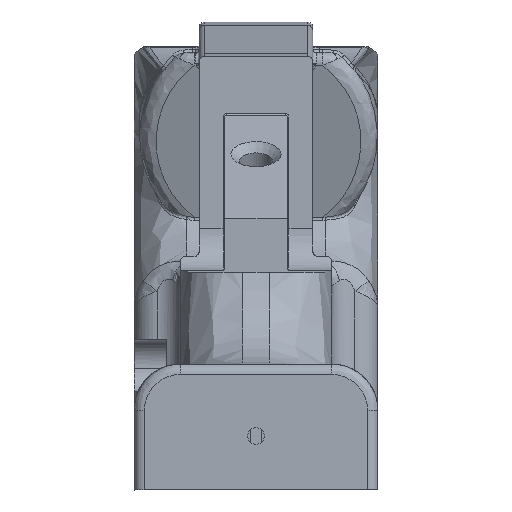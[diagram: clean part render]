
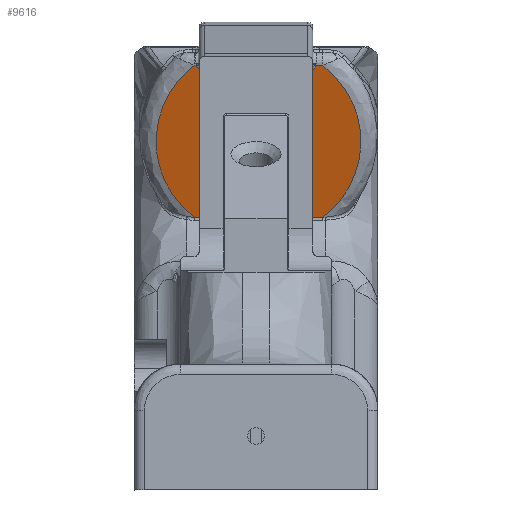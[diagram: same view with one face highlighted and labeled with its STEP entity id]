
A CAD part, left-side view. The second image highlights one B-rep face of the part: STEP entity #9616.
In plain terms, the highlighted face is planar.
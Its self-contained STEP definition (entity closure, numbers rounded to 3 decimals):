
#287 = CARTESIAN_POINT ( 'NONE',  ( -86.38, -58.957, 9.041 ) ) ;
#300 = VERTEX_POINT ( 'NONE', #3083 ) ;
#1211 = EDGE_CURVE ( 'NONE', #7501, #18581, #15948, .T. ) ;
#1220 = ORIENTED_EDGE ( 'NONE', *, *, #18913, .T. ) ;
#1431 = ORIENTED_EDGE ( 'NONE', *, *, #1211, .F. ) ;
#1519 = CARTESIAN_POINT ( 'NONE',  ( -79.11, -35.899, 9.385 ) ) ;
#1531 = CARTESIAN_POINT ( 'NONE',  ( -86.423, -59.093, 9.38 ) ) ;
#1605 = ORIENTED_EDGE ( 'NONE', *, *, #19267, .T. ) ;
#1767 = CARTESIAN_POINT ( 'NONE',  ( -81.144, -42.35, -18.578 ) ) ;
#1839 = ORIENTED_EDGE ( 'NONE', *, *, #10694, .T. ) ;
#1852 = CARTESIAN_POINT ( 'NONE',  ( -86.156, -58.248, 8.376 ) ) ;
#2007 = EDGE_CURVE ( 'NONE', #4205, #10850, #8191, .T. ) ;
#2132 = EDGE_CURVE ( 'NONE', #18581, #7602, #13308, .T. ) ;
#2375 = CARTESIAN_POINT ( 'NONE',  ( -86.342, -58.835, -8.976 ) ) ;
#2548 = B_SPLINE_CURVE_WITH_KNOTS ( 'NONE', 3,
 ( #3280, #13745, #6333, #15331, #7869, #15270, #1852, #18113, #18312, #12299, #3406, #9184, #13610, #13802, #287, #4910 ),
 .UNSPECIFIED., .F., .F.,
 ( 4, 1, 2, 2, 2, 1, 2, 2, 4 ),
 ( 0., 0.125, 0.188, 0.25, 0.5, 0.625, 0.688, 0.75, 1. ),
 .UNSPECIFIED. ) ;
#2953 = CARTESIAN_POINT ( 'NONE',  ( -86.423, -59.093, -3.161 ) ) ;
#3083 = CARTESIAN_POINT ( 'NONE',  ( -79.11, -35.899, -10.166 ) ) ;
#3268 = PLANE ( 'NONE',  #10192 ) ;
#3280 = CARTESIAN_POINT ( 'NONE',  ( -86.122, -58.139, 7.855 ) ) ;
#3406 = CARTESIAN_POINT ( 'NONE',  ( -86.267, -58.6, 8.817 ) ) ;
#3735 = CARTESIAN_POINT ( 'NONE',  ( -86.401, -59.025, -9.062 ) ) ;
#3867 = CARTESIAN_POINT ( 'NONE',  ( -86.191, -58.359, -8.556 ) ) ;
#4205 = VERTEX_POINT ( 'NONE', #8599 ) ;
#4249 = B_SPLINE_CURVE_WITH_KNOTS ( 'NONE', 3,
 ( #8255, #3735, #17134, #2375, #18641, #14331, #8319, #12756, #3867, #5366, #12882, #15653, #14268, #18699, #9691, #8459 ),
 .UNSPECIFIED., .F., .F.,
 ( 4, 1, 2, 2, 2, 1, 2, 2, 4 ),
 ( 0., 0.125, 0.187, 0.25, 0.5, 0.625, 0.687, 0.75, 1. ),
 .UNSPECIFIED. ) ;
#4419 = DIRECTION ( 'NONE',  ( 0., 0., -1. ) ) ;
#4565 = CARTESIAN_POINT ( 'NONE',  ( -86.423, -59.093, -0.39 ) ) ;
#4910 = CARTESIAN_POINT ( 'NONE',  ( -86.423, -59.093, 9.083 ) ) ;
#4961 = VECTOR ( 'NONE', #9032, 1000. ) ;
#5224 = CARTESIAN_POINT ( 'NONE',  ( -86.122, -58.139, -0.39 ) ) ;
#5366 = CARTESIAN_POINT ( 'NONE',  ( -86.173, -58.301, -8.467 ) ) ;
#6333 = CARTESIAN_POINT ( 'NONE',  ( -86.125, -58.147, 8.019 ) ) ;
#7501 = VERTEX_POINT ( 'NONE', #1519 ) ;
#7602 = VERTEX_POINT ( 'NONE', #18106 ) ;
#7869 = CARTESIAN_POINT ( 'NONE',  ( -86.136, -58.184, 8.18 ) ) ;
#8191 = LINE ( 'NONE', #5224, #18701 ) ;
#8206 = LINE ( 'NONE', #2953, #18248 ) ;
#8255 = CARTESIAN_POINT ( 'NONE',  ( -86.423, -59.093, -9.083 ) ) ;
#8319 = CARTESIAN_POINT ( 'NONE',  ( -86.266, -58.595, -8.823 ) ) ;
#8459 = CARTESIAN_POINT ( 'NONE',  ( -86.122, -58.139, -7.855 ) ) ;
#8599 = CARTESIAN_POINT ( 'NONE',  ( -86.122, -58.139, -7.855 ) ) ;
#8964 = EDGE_CURVE ( 'NONE', #11806, #15990, #8206, .T. ) ;
#9032 = DIRECTION ( 'NONE',  ( 0., 0., -1. ) ) ;
#9039 = CARTESIAN_POINT ( 'NONE',  ( -84.39, -52.645, -18.576 ) ) ;
#9184 = CARTESIAN_POINT ( 'NONE',  ( -86.285, -58.657, 8.862 ) ) ;
#9616 = ADVANCED_FACE ( 'NONE', ( #17098 ), #3268, .T. ) ;
#9691 = CARTESIAN_POINT ( 'NONE',  ( -86.122, -58.139, -7.988 ) ) ;
#10192 = AXIS2_PLACEMENT_3D ( 'NONE', #10394, #13596, #13666 ) ;
#10394 = CARTESIAN_POINT ( 'NONE',  ( -82.766, -47.494, -0.39 ) ) ;
#10685 = CARTESIAN_POINT ( 'NONE',  ( -79.11, -35.899, 9.385 ) ) ;
#10694 = EDGE_CURVE ( 'NONE', #10850, #7602, #2548, .T. ) ;
#10850 = VERTEX_POINT ( 'NONE', #12365 ) ;
#10875 = ORIENTED_EDGE ( 'NONE', *, *, #2132, .F. ) ;
#11022 = ORIENTED_EDGE ( 'NONE', *, *, #8964, .F. ) ;
#11806 = VERTEX_POINT ( 'NONE', #16046 ) ;
#12152 = DIRECTION ( 'NONE',  ( 0., 0., -1. ) ) ;
#12255 = CARTESIAN_POINT ( 'NONE',  ( -86.423, -59.093, 9.38 ) ) ;
#12299 = CARTESIAN_POINT ( 'NONE',  ( -86.242, -58.518, 8.747 ) ) ;
#12365 = CARTESIAN_POINT ( 'NONE',  ( -86.122, -58.139, 7.855 ) ) ;
#12509 = ORIENTED_EDGE ( 'NONE', *, *, #2007, .T. ) ;
#12756 = CARTESIAN_POINT ( 'NONE',  ( -86.233, -58.49, -8.725 ) ) ;
#12882 = CARTESIAN_POINT ( 'NONE',  ( -86.159, -58.255, -8.373 ) ) ;
#13308 = LINE ( 'NONE', #4565, #4961 ) ;
#13592 = CARTESIAN_POINT ( 'NONE',  ( -79.11, -35.899, -10.166 ) ) ;
#13596 = DIRECTION ( 'NONE',  ( -0.954, 0.301, 0. ) ) ;
#13610 = CARTESIAN_POINT ( 'NONE',  ( -86.295, -58.688, 8.885 ) ) ;
#13666 = DIRECTION ( 'NONE',  ( -0.301, -0.954, 0. ) ) ;
#13701 = CARTESIAN_POINT ( 'NONE',  ( -84.39, -52.645, 17.795 ) ) ;
#13745 = CARTESIAN_POINT ( 'NONE',  ( -86.122, -58.139, 7.921 ) ) ;
#13786 = CARTESIAN_POINT ( 'NONE',  ( -86.423, -59.093, -10.161 ) ) ;
#13802 = CARTESIAN_POINT ( 'NONE',  ( -86.34, -58.832, 8.982 ) ) ;
#13964 = EDGE_LOOP ( 'NONE', ( #15762, #11022, #1220, #12509, #1839, #10875, #1431, #1605 ) ) ;
#14268 = CARTESIAN_POINT ( 'NONE',  ( -86.146, -58.214, -8.275 ) ) ;
#14331 = CARTESIAN_POINT ( 'NONE',  ( -86.314, -58.747, -8.924 ) ) ;
#14340 = EDGE_CURVE ( 'NONE', #15990, #300, #17252, .T. ) ;
#15270 = CARTESIAN_POINT ( 'NONE',  ( -86.139, -58.192, 8.21 ) ) ;
#15331 = CARTESIAN_POINT ( 'NONE',  ( -86.131, -58.167, 8.116 ) ) ;
#15349 = CARTESIAN_POINT ( 'NONE',  ( -81.144, -42.35, 17.797 ) ) ;
#15653 = CARTESIAN_POINT ( 'NONE',  ( -86.15, -58.227, -8.309 ) ) ;
#15762 = ORIENTED_EDGE ( 'NONE', *, *, #14340, .F. ) ;
#15948 =( BOUNDED_CURVE ( )  B_SPLINE_CURVE ( 3, ( #10685, #15349, #13701, #12255 ),
 .UNSPECIFIED., .F., .T. ) 
 B_SPLINE_CURVE_WITH_KNOTS ( ( 4, 4 ),
 ( 0., 1. ),
 .UNSPECIFIED. ) 
 CURVE ( )  GEOMETRIC_REPRESENTATION_ITEM ( )  RATIONAL_B_SPLINE_CURVE ( ( 1., 0.751, 0.751, 1. ) ) 
 REPRESENTATION_ITEM ( '' )  );
#15990 = VERTEX_POINT ( 'NONE', #18988 ) ;
#16046 = CARTESIAN_POINT ( 'NONE',  ( -86.423, -59.093, -9.083 ) ) ;
#16542 = LINE ( 'NONE', #16602, #16761 ) ;
#16602 = CARTESIAN_POINT ( 'NONE',  ( -79.11, -35.899, -14.288 ) ) ;
#16761 = VECTOR ( 'NONE', #12152, 1000. ) ;
#17098 = FACE_OUTER_BOUND ( 'NONE', #13964, .T. ) ;
#17134 = CARTESIAN_POINT ( 'NONE',  ( -86.371, -58.927, -9.024 ) ) ;
#17252 =( BOUNDED_CURVE ( )  B_SPLINE_CURVE ( 3, ( #13786, #9039, #1767, #13592 ),
 .UNSPECIFIED., .F., .F. ) 
 B_SPLINE_CURVE_WITH_KNOTS ( ( 4, 4 ),
 ( 0., 1. ),
 .UNSPECIFIED. ) 
 CURVE ( )  GEOMETRIC_REPRESENTATION_ITEM ( )  RATIONAL_B_SPLINE_CURVE ( ( 1., 0.751, 0.751, 1. ) ) 
 REPRESENTATION_ITEM ( '' )  );
#18106 = CARTESIAN_POINT ( 'NONE',  ( -86.423, -59.093, 9.083 ) ) ;
#18113 = CARTESIAN_POINT ( 'NONE',  ( -86.178, -58.315, 8.499 ) ) ;
#18248 = VECTOR ( 'NONE', #4419, 1000. ) ;
#18312 = CARTESIAN_POINT ( 'NONE',  ( -86.219, -58.446, 8.669 ) ) ;
#18581 = VERTEX_POINT ( 'NONE', #1531 ) ;
#18641 = CARTESIAN_POINT ( 'NONE',  ( -86.323, -58.775, -8.942 ) ) ;
#18699 = CARTESIAN_POINT ( 'NONE',  ( -86.129, -58.161, -8.117 ) ) ;
#18701 = VECTOR ( 'NONE', #18951, 1000. ) ;
#18913 = EDGE_CURVE ( 'NONE', #11806, #4205, #4249, .T. ) ;
#18951 = DIRECTION ( 'NONE',  ( 0., 0., 1. ) ) ;
#18988 = CARTESIAN_POINT ( 'NONE',  ( -86.423, -59.093, -10.161 ) ) ;
#19267 = EDGE_CURVE ( 'NONE', #7501, #300, #16542, .T. ) ;
